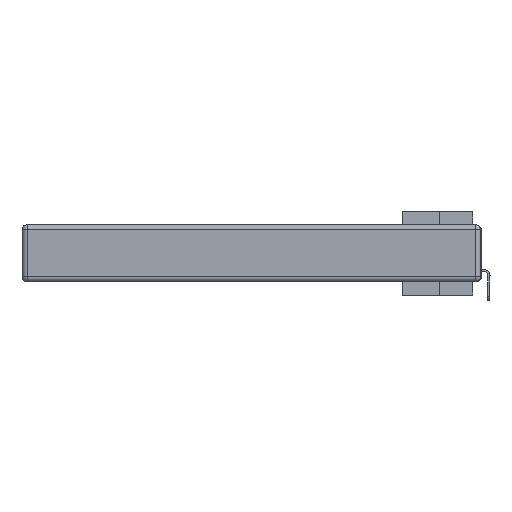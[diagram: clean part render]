
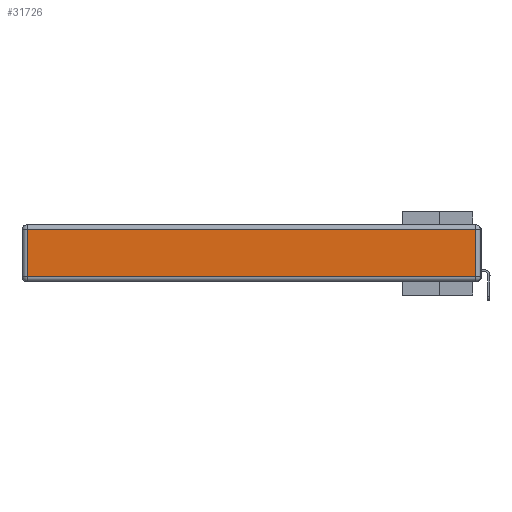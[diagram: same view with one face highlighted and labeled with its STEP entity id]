
A CAD part, left-side view. The second image highlights one B-rep face of the part: STEP entity #31726.
In plain terms, the highlighted planar face has unit normal (-1, 0, 0).
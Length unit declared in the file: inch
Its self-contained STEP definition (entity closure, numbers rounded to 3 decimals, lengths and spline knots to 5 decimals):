
#607 = CARTESIAN_POINT ( 'NONE',  ( 0., 2.72, -0.03 ) ) ;
#1806 = CARTESIAN_POINT ( 'NONE',  ( 0., 2.72, -0.313 ) ) ;
#2270 = ORIENTED_EDGE ( 'NONE', *, *, #19897, .T. ) ;
#3222 = DIRECTION ( 'NONE',  ( 0., 0., -1. ) ) ;
#3496 = EDGE_LOOP ( 'NONE', ( #4593, #33894, #2270, #5600 ) ) ;
#4371 = CARTESIAN_POINT ( 'NONE',  ( 0., 0.03, -0.03 ) ) ;
#4593 = ORIENTED_EDGE ( 'NONE', *, *, #31401, .T. ) ;
#5493 = CARTESIAN_POINT ( 'NONE',  ( 0., 0.03, -0.313 ) ) ;
#5600 = ORIENTED_EDGE ( 'NONE', *, *, #23130, .T. ) ;
#5862 = CARTESIAN_POINT ( 'NONE',  ( 0., 2.72, -0.343 ) ) ;
#6655 = LINE ( 'NONE', #33340, #28163 ) ;
#8212 = FACE_OUTER_BOUND ( 'NONE', #3496, .T. ) ;
#11800 = VECTOR ( 'NONE', #18547, 39.37008 ) ;
#13979 = VECTOR ( 'NONE', #21545, 39.37008 ) ;
#15355 = CARTESIAN_POINT ( 'NONE',  ( 0., 0., -0.343 ) ) ;
#15527 = PLANE ( 'NONE',  #29656 ) ;
#18547 = DIRECTION ( 'NONE',  ( 0., -1., 0. ) ) ;
#19897 = EDGE_CURVE ( 'NONE', #25913, #21910, #6655, .T. ) ;
#20565 = VERTEX_POINT ( 'NONE', #5493 ) ;
#21197 = CARTESIAN_POINT ( 'NONE',  ( 0., 0.03, -0.343 ) ) ;
#21284 = DIRECTION ( 'NONE',  ( -1., 0., 0. ) ) ;
#21545 = DIRECTION ( 'NONE',  ( 0., 0., 1. ) ) ;
#21910 = VERTEX_POINT ( 'NONE', #607 ) ;
#23130 = EDGE_CURVE ( 'NONE', #21910, #23426, #29235, .T. ) ;
#23426 = VERTEX_POINT ( 'NONE', #1806 ) ;
#23438 = LINE ( 'NONE', #26898, #11800 ) ;
#23799 = VECTOR ( 'NONE', #3222, 39.37008 ) ;
#25913 = VERTEX_POINT ( 'NONE', #4371 ) ;
#26179 = DIRECTION ( 'NONE',  ( 0., 0., 1. ) ) ;
#26898 = CARTESIAN_POINT ( 'NONE',  ( 0., 0., -0.313 ) ) ;
#28163 = VECTOR ( 'NONE', #30892, 39.37008 ) ;
#29036 = LINE ( 'NONE', #21197, #13979 ) ;
#29235 = LINE ( 'NONE', #5862, #23799 ) ;
#29656 = AXIS2_PLACEMENT_3D ( 'NONE', #15355, #21284, #26179 ) ;
#29665 = EDGE_CURVE ( 'NONE', #20565, #25913, #29036, .T. ) ;
#30892 = DIRECTION ( 'NONE',  ( 0., 1., 0. ) ) ;
#31401 = EDGE_CURVE ( 'NONE', #23426, #20565, #23438, .T. ) ;
#31726 = ADVANCED_FACE ( 'NONE', ( #8212 ), #15527, .T. ) ;
#33340 = CARTESIAN_POINT ( 'NONE',  ( 0., 2.75, -0.03 ) ) ;
#33894 = ORIENTED_EDGE ( 'NONE', *, *, #29665, .T. ) ;
